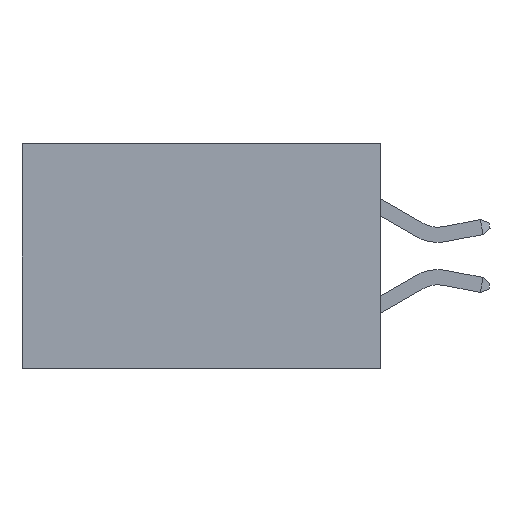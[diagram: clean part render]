
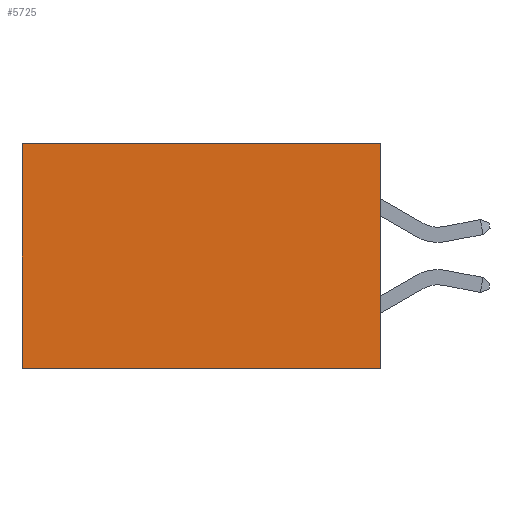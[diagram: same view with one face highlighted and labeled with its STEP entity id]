
A CAD part, left-side view. The second image highlights one B-rep face of the part: STEP entity #5725.
In plain terms, the highlighted planar face has unit normal (-1, 0, 0).
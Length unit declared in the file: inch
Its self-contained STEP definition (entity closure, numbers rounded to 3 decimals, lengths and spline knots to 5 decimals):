
#526 = ORIENTED_EDGE ( 'NONE', *, *, #10625, .F. ) ;
#626 = LINE ( 'NONE', #20806, #17855 ) ;
#690 = LINE ( 'NONE', #15832, #4796 ) ;
#2050 = CARTESIAN_POINT ( 'NONE',  ( 0.277, 0., -0.37 ) ) ;
#2125 = EDGE_CURVE ( 'NONE', #17204, #6469, #2424, .T. ) ;
#2424 = LINE ( 'NONE', #12916, #20135 ) ;
#2978 = DIRECTION ( 'NONE',  ( 0., 1., 0. ) ) ;
#3480 = AXIS2_PLACEMENT_3D ( 'NONE', #7901, #7754, #7638 ) ;
#3948 = CARTESIAN_POINT ( 'NONE',  ( 0.277, 0., 0. ) ) ;
#4796 = VECTOR ( 'NONE', #7409, 39.37008 ) ;
#5725 = ADVANCED_FACE ( 'NONE', ( #19149 ), #8894, .F. ) ;
#5947 = ORIENTED_EDGE ( 'NONE', *, *, #9256, .T. ) ;
#6071 = VERTEX_POINT ( 'NONE', #17367 ) ;
#6469 = VERTEX_POINT ( 'NONE', #2050 ) ;
#7409 = DIRECTION ( 'NONE',  ( 0., 0., -1. ) ) ;
#7638 = DIRECTION ( 'NONE',  ( 0., 0., -1. ) ) ;
#7747 = CARTESIAN_POINT ( 'NONE',  ( 0.277, 0.59, 0. ) ) ;
#7754 = DIRECTION ( 'NONE',  ( 1., 0., 0. ) ) ;
#7901 = CARTESIAN_POINT ( 'NONE',  ( 0.277, 0., -0.37 ) ) ;
#8894 = PLANE ( 'NONE',  #3480 ) ;
#9256 = EDGE_CURVE ( 'NONE', #17320, #6071, #690, .T. ) ;
#10625 = EDGE_CURVE ( 'NONE', #6469, #6071, #626, .T. ) ;
#11428 = DIRECTION ( 'NONE',  ( 0., 0., -1. ) ) ;
#11645 = CARTESIAN_POINT ( 'NONE',  ( 0.277, 0., 0. ) ) ;
#12373 = DIRECTION ( 'NONE',  ( 0., 1., 0. ) ) ;
#12916 = CARTESIAN_POINT ( 'NONE',  ( 0.277, 0., -0.37 ) ) ;
#14073 = ORIENTED_EDGE ( 'NONE', *, *, #20528, .T. ) ;
#14724 = LINE ( 'NONE', #11645, #15251 ) ;
#14880 = ORIENTED_EDGE ( 'NONE', *, *, #2125, .F. ) ;
#15251 = VECTOR ( 'NONE', #2978, 39.37008 ) ;
#15832 = CARTESIAN_POINT ( 'NONE',  ( 0.277, 0.59, -0.37 ) ) ;
#16535 = EDGE_LOOP ( 'NONE', ( #5947, #526, #14880, #14073 ) ) ;
#17204 = VERTEX_POINT ( 'NONE', #3948 ) ;
#17320 = VERTEX_POINT ( 'NONE', #7747 ) ;
#17367 = CARTESIAN_POINT ( 'NONE',  ( 0.277, 0.59, -0.37 ) ) ;
#17855 = VECTOR ( 'NONE', #12373, 39.37008 ) ;
#19149 = FACE_OUTER_BOUND ( 'NONE', #16535, .T. ) ;
#20135 = VECTOR ( 'NONE', #11428, 39.37008 ) ;
#20528 = EDGE_CURVE ( 'NONE', #17204, #17320, #14724, .T. ) ;
#20806 = CARTESIAN_POINT ( 'NONE',  ( 0.277, 0., -0.37 ) ) ;
